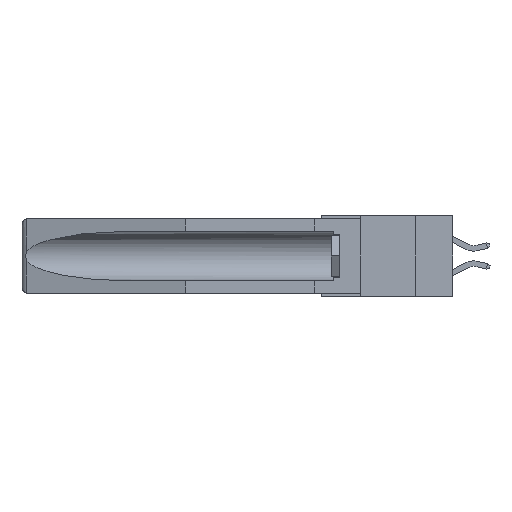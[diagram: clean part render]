
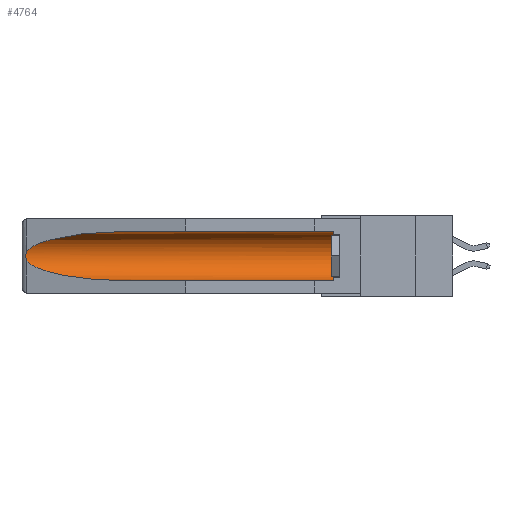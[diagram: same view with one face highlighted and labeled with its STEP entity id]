
A CAD part, left-side view. The second image highlights one B-rep face of the part: STEP entity #4764.
In plain terms, the highlighted cylindrical face has radius 2.857 mm (diameter 5.715 mm), a partial arc.
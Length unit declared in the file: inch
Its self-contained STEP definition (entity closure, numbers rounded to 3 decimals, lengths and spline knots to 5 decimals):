
#765 = LINE ( 'NONE', #11351, #14884 ) ;
#776 = ORIENTED_EDGE ( 'NONE', *, *, #12356, .F. ) ;
#1463 = ORIENTED_EDGE ( 'NONE', *, *, #13194, .T. ) ;
#1836 = CARTESIAN_POINT ( 'NONE',  ( 0.155, 0.126, -0.284 ) ) ;
#2160 = CARTESIAN_POINT ( 'NONE',  ( 0.26597, 1.5296, -0.19026 ) ) ;
#2181 = FACE_OUTER_BOUND ( 'NONE', #6565, .T. ) ;
#2600 = EDGE_CURVE ( 'NONE', #15867, #10403, #765, .T. ) ;
#3209 = CARTESIAN_POINT ( 'NONE',  ( 0.26597, 1.52961, -0.15275 ) ) ;
#3260 = EDGE_CURVE ( 'NONE', #6791, #5930, #14092, .T. ) ;
#3795 = DIRECTION ( 'NONE',  ( 0., 1., 0. ) ) ;
#4173 = ORIENTED_EDGE ( 'NONE', *, *, #10579, .T. ) ;
#4282 = CARTESIAN_POINT ( 'NONE',  ( 0.2675, 1.53308, -0.17534 ) ) ;
#4764 = ADVANCED_FACE ( 'NONE', ( #2181 ), #14810, .F. ) ;
#4955 = CARTESIAN_POINT ( 'NONE',  ( 0.155, 1.07973, -0.284 ) ) ;
#4996 = CARTESIAN_POINT ( 'NONE',  ( 0.155, 1.07973, -0.059 ) ) ;
#5601 = CARTESIAN_POINT ( 'NONE',  ( 0.155, -0.30754, -0.1715 ) ) ;
#5667 = DIRECTION ( 'NONE',  ( 0., 0., 1. ) ) ;
#5930 = VERTEX_POINT ( 'NONE', #14978 ) ;
#6551 = EDGE_CURVE ( 'NONE', #5930, #7696, #11224, .T. ) ;
#6565 = EDGE_LOOP ( 'NONE', ( #1463, #13344, #13371, #776, #4173, #10864 ) ) ;
#6609 = CARTESIAN_POINT ( 'NONE',  ( 0.26537, 1.52718, -0.14972 ) ) ;
#6757 = CARTESIAN_POINT ( 'NONE',  ( 0.26654, 1.53092, -0.15636 ) ) ;
#6791 = VERTEX_POINT ( 'NONE', #13172 ) ;
#6920 = CARTESIAN_POINT ( 'NONE',  ( 0.26537, 1.52718, -0.14972 ) ) ;
#7335 = VERTEX_POINT ( 'NONE', #1836 ) ;
#7556 = VECTOR ( 'NONE', #10680, 39.37008 ) ;
#7641 = CARTESIAN_POINT ( 'NONE',  ( 0.26537, 1.52718, -0.19328 ) ) ;
#7696 = VERTEX_POINT ( 'NONE', #9850 ) ;
#7769 = CARTESIAN_POINT ( 'NONE',  ( 0.155, 0.126, -0.1715 ) ) ;
#7945 = CARTESIAN_POINT ( 'NONE',  ( 0.2673, 1.53269, -0.17917 ) ) ;
#8140 = CARTESIAN_POINT ( 'NONE',  ( 0.155, -0.30754, -0.284 ) ) ;
#8816 = CARTESIAN_POINT ( 'NONE',  ( 0.25451, 1.48313, -0.24835 ) ) ;
#9368 = CARTESIAN_POINT ( 'NONE',  ( 0.155, 0.126, -0.059 ) ) ;
#9850 = CARTESIAN_POINT ( 'NONE',  ( 0.155, 1.07973, -0.284 ) ) ;
#9866 = AXIS2_PLACEMENT_3D ( 'NONE', #7769, #12843, #5667 ) ;
#10199 = CIRCLE ( 'NONE', #9866, 0.1125 ) ;
#10403 = VERTEX_POINT ( 'NONE', #4996 ) ;
#10543 = CARTESIAN_POINT ( 'NONE',  ( 0.2675, 1.53308, -0.16763 ) ) ;
#10579 = EDGE_CURVE ( 'NONE', #7335, #15867, #10199, .T. ) ;
#10680 = DIRECTION ( 'NONE',  ( 0., 1., 0. ) ) ;
#10864 = ORIENTED_EDGE ( 'NONE', *, *, #2600, .T. ) ;
#11203 = CARTESIAN_POINT ( 'NONE',  ( 0.21114, 1.30732, -0.284 ) ) ;
#11224 =( BOUNDED_CURVE ( )  B_SPLINE_CURVE ( 3, ( #7641, #8816, #11203, #4955 ),
 .UNSPECIFIED., .F., .T. ) 
 B_SPLINE_CURVE_WITH_KNOTS ( ( 4, 4 ),
 ( 0.1948, 1.5708 ),
 .UNSPECIFIED. ) 
 CURVE ( )  GEOMETRIC_REPRESENTATION_ITEM ( )  RATIONAL_B_SPLINE_CURVE ( ( 1., 0.848, 0.848, 1. ) ) 
 REPRESENTATION_ITEM ( '' )  );
#11351 = CARTESIAN_POINT ( 'NONE',  ( 0.155, -0.30754, -0.059 ) ) ;
#11566 = AXIS2_PLACEMENT_3D ( 'NONE', #5601, #14297, #15548 ) ;
#11682 = LINE ( 'NONE', #8140, #7556 ) ;
#11855 = CARTESIAN_POINT ( 'NONE',  ( 0.21114, 1.30732, -0.059 ) ) ;
#11953 = CARTESIAN_POINT ( 'NONE',  ( 0.2673, 1.5327, -0.16383 ) ) ;
#12356 = EDGE_CURVE ( 'NONE', #7335, #7696, #11682, .T. ) ;
#12843 = DIRECTION ( 'NONE',  ( 0., -1., 0. ) ) ;
#12969 = CARTESIAN_POINT ( 'NONE',  ( 0.25451, 1.48313, -0.09465 ) ) ;
#13172 = CARTESIAN_POINT ( 'NONE',  ( 0.26537, 1.52718, -0.14972 ) ) ;
#13194 = EDGE_CURVE ( 'NONE', #10403, #6791, #15065, .T. ) ;
#13265 = CARTESIAN_POINT ( 'NONE',  ( 0.26655, 1.53094, -0.18657 ) ) ;
#13344 = ORIENTED_EDGE ( 'NONE', *, *, #3260, .T. ) ;
#13371 = ORIENTED_EDGE ( 'NONE', *, *, #6551, .T. ) ;
#14092 = B_SPLINE_CURVE_WITH_KNOTS ( 'NONE', 3,
 ( #6920, #3209, #6757, #11953, #10543, #4282, #7945, #13265, #2160, #15076 ),
 .UNSPECIFIED., .F., .F.,
 ( 4, 2, 2, 2, 4 ),
 ( 0., 0.00029, 0.00058, 0.00087, 0.00117 ),
 .UNSPECIFIED. ) ;
#14297 = DIRECTION ( 'NONE',  ( 0., 1., 0. ) ) ;
#14810 = CYLINDRICAL_SURFACE ( 'NONE', #11566, 0.1125 ) ;
#14884 = VECTOR ( 'NONE', #3795, 39.37008 ) ;
#14978 = CARTESIAN_POINT ( 'NONE',  ( 0.26537, 1.52718, -0.19328 ) ) ;
#15065 =( BOUNDED_CURVE ( )  B_SPLINE_CURVE ( 3, ( #15337, #11855, #12969, #6609 ),
 .UNSPECIFIED., .F., .F. ) 
 B_SPLINE_CURVE_WITH_KNOTS ( ( 4, 4 ),
 ( 4.71239, 6.08839 ),
 .UNSPECIFIED. ) 
 CURVE ( )  GEOMETRIC_REPRESENTATION_ITEM ( )  RATIONAL_B_SPLINE_CURVE ( ( 1., 0.848, 0.848, 1. ) ) 
 REPRESENTATION_ITEM ( '' )  );
#15076 = CARTESIAN_POINT ( 'NONE',  ( 0.26537, 1.52718, -0.19328 ) ) ;
#15337 = CARTESIAN_POINT ( 'NONE',  ( 0.155, 1.07973, -0.059 ) ) ;
#15548 = DIRECTION ( 'NONE',  ( 0., 0., 1. ) ) ;
#15867 = VERTEX_POINT ( 'NONE', #9368 ) ;
